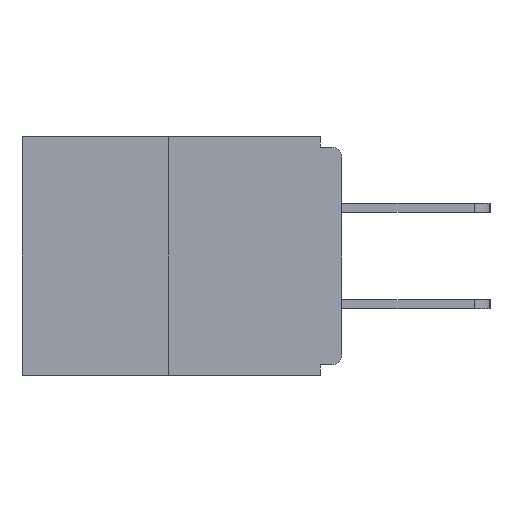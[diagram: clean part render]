
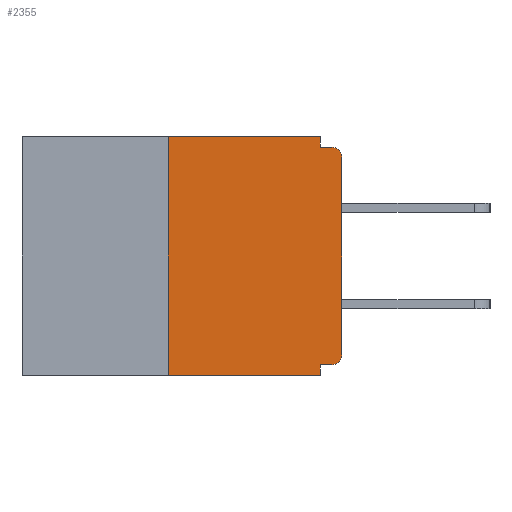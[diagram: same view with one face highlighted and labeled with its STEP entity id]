
A CAD part, left-side view. The second image highlights one B-rep face of the part: STEP entity #2355.
In plain terms, the highlighted planar face has unit normal (-1, 0, 0).
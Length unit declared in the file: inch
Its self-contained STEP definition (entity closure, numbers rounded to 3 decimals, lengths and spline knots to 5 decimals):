
#259 = ORIENTED_EDGE ( 'NONE', *, *, #2937, .F. ) ;
#1735 = EDGE_CURVE ( 'NONE', #13309, #4436, #2118, .T. ) ;
#1959 = LINE ( 'NONE', #12689, #7243 ) ;
#2118 = LINE ( 'NONE', #14479, #11989 ) ;
#2355 = ADVANCED_FACE ( 'NONE', ( #3383 ), #4805, .F. ) ;
#2869 = DIRECTION ( 'NONE',  ( -1., 0., 0. ) ) ;
#2937 = EDGE_CURVE ( 'NONE', #4436, #14092, #1959, .T. ) ;
#3186 = EDGE_LOOP ( 'NONE', ( #11773, #8771, #13605, #15454, #13260, #5785, #10688, #19699, #259, #6892 ) ) ;
#3383 = FACE_OUTER_BOUND ( 'NONE', #3186, .T. ) ;
#3459 = EDGE_CURVE ( 'NONE', #18013, #4018, #13493, .T. ) ;
#3726 = LINE ( 'NONE', #3833, #17953 ) ;
#3821 = VERTEX_POINT ( 'NONE', #12549 ) ;
#3833 = CARTESIAN_POINT ( 'NONE',  ( 0., 0.25, 0. ) ) ;
#4018 = VERTEX_POINT ( 'NONE', #13841 ) ;
#4118 = AXIS2_PLACEMENT_3D ( 'NONE', #8758, #8655, #19456 ) ;
#4154 = VERTEX_POINT ( 'NONE', #14208 ) ;
#4358 = LINE ( 'NONE', #7323, #11847 ) ;
#4436 = VERTEX_POINT ( 'NONE', #15498 ) ;
#4667 = EDGE_CURVE ( 'NONE', #12740, #4154, #12671, .T. ) ;
#4773 = CIRCLE ( 'NONE', #8333, 0.015 ) ;
#4805 = PLANE ( 'NONE',  #17243 ) ;
#5467 = LINE ( 'NONE', #7203, #8528 ) ;
#5785 = ORIENTED_EDGE ( 'NONE', *, *, #16116, .T. ) ;
#6163 = DIRECTION ( 'NONE',  ( 0., -1., 0. ) ) ;
#6892 = ORIENTED_EDGE ( 'NONE', *, *, #1735, .F. ) ;
#7102 = EDGE_CURVE ( 'NONE', #3821, #13309, #10696, .T. ) ;
#7113 = CARTESIAN_POINT ( 'NONE',  ( 0., 0., 0. ) ) ;
#7203 = CARTESIAN_POINT ( 'NONE',  ( 0., 0., -0.328 ) ) ;
#7243 = VECTOR ( 'NONE', #8110, 39.37008 ) ;
#7323 = CARTESIAN_POINT ( 'NONE',  ( 0., 0.031, -0.343 ) ) ;
#8110 = DIRECTION ( 'NONE',  ( 0., -1., 0. ) ) ;
#8333 = AXIS2_PLACEMENT_3D ( 'NONE', #12447, #2869, #15121 ) ;
#8528 = VECTOR ( 'NONE', #11588, 39.37008 ) ;
#8574 = DIRECTION ( 'NONE',  ( 0., 0., 1. ) ) ;
#8655 = DIRECTION ( 'NONE',  ( -1., 0., 0. ) ) ;
#8758 = CARTESIAN_POINT ( 'NONE',  ( 0., 0.015, -0.03 ) ) ;
#8771 = ORIENTED_EDGE ( 'NONE', *, *, #16364, .F. ) ;
#9704 = VERTEX_POINT ( 'NONE', #10006 ) ;
#10006 = CARTESIAN_POINT ( 'NONE',  ( 0., 0.031, -0.328 ) ) ;
#10315 = CARTESIAN_POINT ( 'NONE',  ( 0., 0.25, -0.343 ) ) ;
#10688 = ORIENTED_EDGE ( 'NONE', *, *, #3459, .T. ) ;
#10696 = LINE ( 'NONE', #16771, #19337 ) ;
#10719 = CARTESIAN_POINT ( 'NONE',  ( 0., 0.015, -0.015 ) ) ;
#11588 = DIRECTION ( 'NONE',  ( 0., 1., 0. ) ) ;
#11773 = ORIENTED_EDGE ( 'NONE', *, *, #7102, .F. ) ;
#11847 = VECTOR ( 'NONE', #16704, 39.37008 ) ;
#11849 = CARTESIAN_POINT ( 'NONE',  ( 0., 0., -0.313 ) ) ;
#11989 = VECTOR ( 'NONE', #17785, 39.37008 ) ;
#12447 = CARTESIAN_POINT ( 'NONE',  ( 0., 0.015, -0.313 ) ) ;
#12515 = CARTESIAN_POINT ( 'NONE',  ( 0., 0.46, 0. ) ) ;
#12549 = CARTESIAN_POINT ( 'NONE',  ( 0., 0.25, 0. ) ) ;
#12671 = LINE ( 'NONE', #17306, #18110 ) ;
#12689 = CARTESIAN_POINT ( 'NONE',  ( 0., 0., -0.015 ) ) ;
#12740 = VERTEX_POINT ( 'NONE', #10315 ) ;
#12984 = CARTESIAN_POINT ( 'NONE',  ( 0., 0.015, -0.328 ) ) ;
#13260 = ORIENTED_EDGE ( 'NONE', *, *, #14605, .F. ) ;
#13309 = VERTEX_POINT ( 'NONE', #16948 ) ;
#13493 = LINE ( 'NONE', #7113, #14490 ) ;
#13522 = EDGE_CURVE ( 'NONE', #4018, #14092, #15661, .T. ) ;
#13605 = ORIENTED_EDGE ( 'NONE', *, *, #4667, .T. ) ;
#13841 = CARTESIAN_POINT ( 'NONE',  ( 0., 0., -0.03 ) ) ;
#14092 = VERTEX_POINT ( 'NONE', #10719 ) ;
#14101 = EDGE_CURVE ( 'NONE', #9704, #4154, #4358, .T. ) ;
#14208 = CARTESIAN_POINT ( 'NONE',  ( 0., 0.031, -0.343 ) ) ;
#14479 = CARTESIAN_POINT ( 'NONE',  ( 0., 0.031, 0. ) ) ;
#14490 = VECTOR ( 'NONE', #17918, 39.37008 ) ;
#14582 = VERTEX_POINT ( 'NONE', #12984 ) ;
#14605 = EDGE_CURVE ( 'NONE', #14582, #9704, #5467, .T. ) ;
#15121 = DIRECTION ( 'NONE',  ( 0., 0., -1. ) ) ;
#15454 = ORIENTED_EDGE ( 'NONE', *, *, #14101, .F. ) ;
#15498 = CARTESIAN_POINT ( 'NONE',  ( 0., 0.031, -0.015 ) ) ;
#15661 = CIRCLE ( 'NONE', #4118, 0.015 ) ;
#16116 = EDGE_CURVE ( 'NONE', #14582, #18013, #4773, .T. ) ;
#16364 = EDGE_CURVE ( 'NONE', #12740, #3821, #3726, .T. ) ;
#16704 = DIRECTION ( 'NONE',  ( 0., 0., -1. ) ) ;
#16771 = CARTESIAN_POINT ( 'NONE',  ( 0., 0.46, 0. ) ) ;
#16948 = CARTESIAN_POINT ( 'NONE',  ( 0., 0.031, 0. ) ) ;
#17243 = AXIS2_PLACEMENT_3D ( 'NONE', #12515, #18479, #18680 ) ;
#17306 = CARTESIAN_POINT ( 'NONE',  ( 0., 0.46, -0.343 ) ) ;
#17785 = DIRECTION ( 'NONE',  ( 0., 0., -1. ) ) ;
#17918 = DIRECTION ( 'NONE',  ( 0., 0., 1. ) ) ;
#17953 = VECTOR ( 'NONE', #8574, 39.37008 ) ;
#18013 = VERTEX_POINT ( 'NONE', #11849 ) ;
#18110 = VECTOR ( 'NONE', #18834, 39.37008 ) ;
#18479 = DIRECTION ( 'NONE',  ( 1., 0., 0. ) ) ;
#18680 = DIRECTION ( 'NONE',  ( 0., 0., -1. ) ) ;
#18834 = DIRECTION ( 'NONE',  ( 0., -1., 0. ) ) ;
#19337 = VECTOR ( 'NONE', #6163, 39.37008 ) ;
#19456 = DIRECTION ( 'NONE',  ( 0., 0., -1. ) ) ;
#19699 = ORIENTED_EDGE ( 'NONE', *, *, #13522, .T. ) ;
